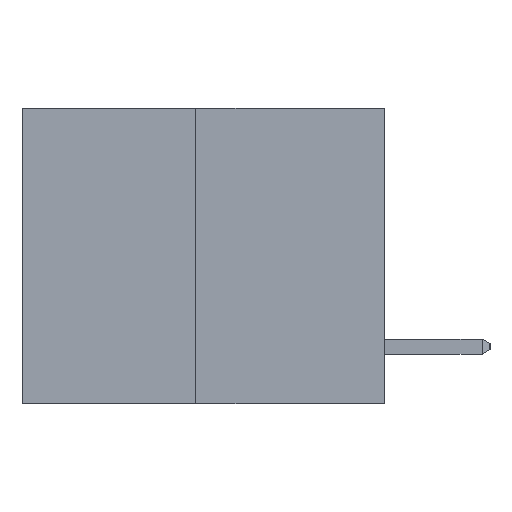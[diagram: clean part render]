
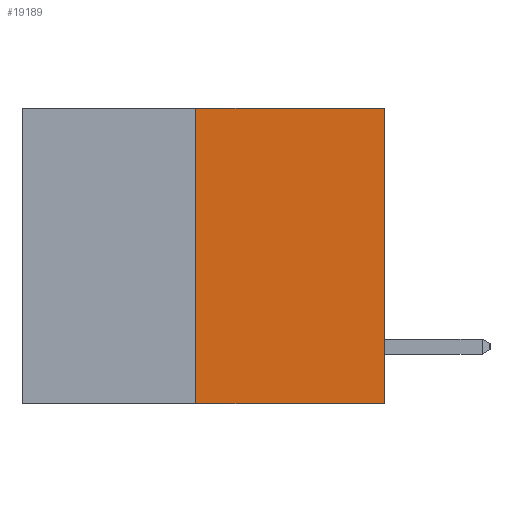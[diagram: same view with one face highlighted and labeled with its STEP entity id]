
A CAD part, left-side view. The second image highlights one B-rep face of the part: STEP entity #19189.
In plain terms, the highlighted planar face has unit normal (-1, 0, 0).
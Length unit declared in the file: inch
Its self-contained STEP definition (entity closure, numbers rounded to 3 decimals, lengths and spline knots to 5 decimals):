
#54 = LINE ( 'NONE', #17943, #2688 ) ;
#218 = CARTESIAN_POINT ( 'NONE',  ( 0., 0.6, 0. ) ) ;
#2688 = VECTOR ( 'NONE', #19963, 39.37008 ) ;
#3870 = VERTEX_POINT ( 'NONE', #5976 ) ;
#4580 = VERTEX_POINT ( 'NONE', #17502 ) ;
#4626 = DIRECTION ( 'NONE',  ( 1., 0., 0. ) ) ;
#5650 = FACE_OUTER_BOUND ( 'NONE', #8768, .T. ) ;
#5976 = CARTESIAN_POINT ( 'NONE',  ( 0., 0., 0. ) ) ;
#6293 = VECTOR ( 'NONE', #10698, 39.37008 ) ;
#6398 = VERTEX_POINT ( 'NONE', #14803 ) ;
#6605 = DIRECTION ( 'NONE',  ( 0., -1., 0. ) ) ;
#6733 = DIRECTION ( 'NONE',  ( 0., 0., -1. ) ) ;
#7845 = VECTOR ( 'NONE', #9021, 39.37008 ) ;
#8546 = CARTESIAN_POINT ( 'NONE',  ( 0., 0.6, -0.49 ) ) ;
#8768 = EDGE_LOOP ( 'NONE', ( #26586, #20391, #13080, #20626 ) ) ;
#9021 = DIRECTION ( 'NONE',  ( 0., 0., 1. ) ) ;
#10127 = VECTOR ( 'NONE', #6605, 39.37008 ) ;
#10698 = DIRECTION ( 'NONE',  ( 0., 0., 1. ) ) ;
#13080 = ORIENTED_EDGE ( 'NONE', *, *, #17633, .T. ) ;
#14803 = CARTESIAN_POINT ( 'NONE',  ( 0., 0.312, 0. ) ) ;
#15721 = LINE ( 'NONE', #8546, #10127 ) ;
#15733 = VERTEX_POINT ( 'NONE', #20433 ) ;
#17287 = PLANE ( 'NONE',  #24048 ) ;
#17502 = CARTESIAN_POINT ( 'NONE',  ( 0., 0., -0.49 ) ) ;
#17633 = EDGE_CURVE ( 'NONE', #4580, #3870, #19110, .T. ) ;
#17943 = CARTESIAN_POINT ( 'NONE',  ( 0., 0.6, 0. ) ) ;
#18209 = LINE ( 'NONE', #23367, #6293 ) ;
#19110 = LINE ( 'NONE', #19731, #7845 ) ;
#19189 = ADVANCED_FACE ( 'NONE', ( #5650 ), #17287, .F. ) ;
#19731 = CARTESIAN_POINT ( 'NONE',  ( 0., 0., 0. ) ) ;
#19766 = EDGE_CURVE ( 'NONE', #15733, #6398, #18209, .T. ) ;
#19963 = DIRECTION ( 'NONE',  ( 0., -1., 0. ) ) ;
#20391 = ORIENTED_EDGE ( 'NONE', *, *, #22221, .T. ) ;
#20433 = CARTESIAN_POINT ( 'NONE',  ( 0., 0.312, -0.49 ) ) ;
#20626 = ORIENTED_EDGE ( 'NONE', *, *, #25962, .F. ) ;
#22221 = EDGE_CURVE ( 'NONE', #15733, #4580, #15721, .T. ) ;
#23367 = CARTESIAN_POINT ( 'NONE',  ( 0., 0.312, -0.49 ) ) ;
#24048 = AXIS2_PLACEMENT_3D ( 'NONE', #218, #4626, #6733 ) ;
#25962 = EDGE_CURVE ( 'NONE', #6398, #3870, #54, .T. ) ;
#26586 = ORIENTED_EDGE ( 'NONE', *, *, #19766, .F. ) ;
